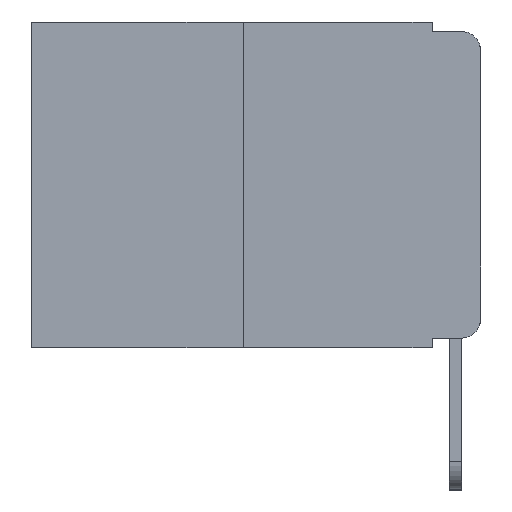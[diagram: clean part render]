
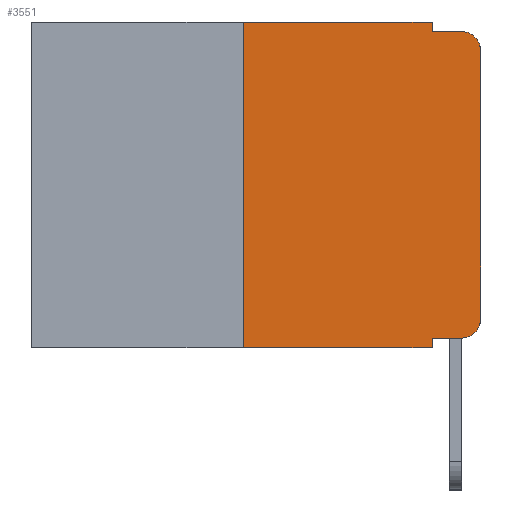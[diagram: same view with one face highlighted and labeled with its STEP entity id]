
A CAD part, left-side view. The second image highlights one B-rep face of the part: STEP entity #3551.
In plain terms, the highlighted planar face has unit normal (-1, 0, 0).
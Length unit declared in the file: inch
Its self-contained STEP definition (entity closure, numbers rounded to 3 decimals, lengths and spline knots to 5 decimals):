
#329 = CIRCLE ( 'NONE', #6323, 0.02 ) ;
#374 = VERTEX_POINT ( 'NONE', #1727 ) ;
#385 = EDGE_CURVE ( 'NONE', #7843, #9507, #11216, .T. ) ;
#397 = EDGE_CURVE ( 'NONE', #10086, #11016, #1003, .T. ) ;
#513 = EDGE_CURVE ( 'NONE', #4225, #12051, #2888, .T. ) ;
#934 = CARTESIAN_POINT ( 'NONE',  ( 0., 0.473, 0. ) ) ;
#1003 = LINE ( 'NONE', #11407, #8877 ) ;
#1082 = CARTESIAN_POINT ( 'NONE',  ( 0., 0.051, -0.333 ) ) ;
#1257 = CARTESIAN_POINT ( 'NONE',  ( 0., 0.25, 0. ) ) ;
#1320 = DIRECTION ( 'NONE',  ( 0., -1., 0. ) ) ;
#1373 = ORIENTED_EDGE ( 'NONE', *, *, #12733, .F. ) ;
#1403 = CARTESIAN_POINT ( 'NONE',  ( 0., 0.25, -0.343 ) ) ;
#1406 = VECTOR ( 'NONE', #1320, 39.37008 ) ;
#1475 = EDGE_CURVE ( 'NONE', #6086, #6269, #4521, .T. ) ;
#1726 = CARTESIAN_POINT ( 'NONE',  ( 0., 0.02, -0.313 ) ) ;
#1727 = CARTESIAN_POINT ( 'NONE',  ( 0., 0., -0.313 ) ) ;
#1803 = DIRECTION ( 'NONE',  ( 0., -1., 0. ) ) ;
#1959 = CARTESIAN_POINT ( 'NONE',  ( 0., 0.051, 0. ) ) ;
#2044 = ORIENTED_EDGE ( 'NONE', *, *, #513, .F. ) ;
#2200 = EDGE_CURVE ( 'NONE', #374, #6086, #4345, .T. ) ;
#2571 = DIRECTION ( 'NONE',  ( 0., 0., -1. ) ) ;
#2708 = DIRECTION ( 'NONE',  ( 0., 0., 1. ) ) ;
#2744 = ORIENTED_EDGE ( 'NONE', *, *, #4756, .F. ) ;
#2835 = DIRECTION ( 'NONE',  ( 0., 0., -1. ) ) ;
#2888 = LINE ( 'NONE', #11461, #12442 ) ;
#2893 = VERTEX_POINT ( 'NONE', #5303 ) ;
#3018 = CARTESIAN_POINT ( 'NONE',  ( 0., 0.02, -0.01 ) ) ;
#3077 = ORIENTED_EDGE ( 'NONE', *, *, #385, .T. ) ;
#3533 = LINE ( 'NONE', #1257, #8553 ) ;
#3551 = ADVANCED_FACE ( 'NONE', ( #6378 ), #11992, .F. ) ;
#4225 = VERTEX_POINT ( 'NONE', #11746 ) ;
#4344 = CARTESIAN_POINT ( 'NONE',  ( 0., 0.051, -0.333 ) ) ;
#4345 = LINE ( 'NONE', #6865, #11883 ) ;
#4492 = CARTESIAN_POINT ( 'NONE',  ( 0., 0.051, 0. ) ) ;
#4521 = CIRCLE ( 'NONE', #12044, 0.02 ) ;
#4611 = DIRECTION ( 'NONE',  ( 1., 0., 0. ) ) ;
#4756 = EDGE_CURVE ( 'NONE', #7843, #11016, #8027, .T. ) ;
#4771 = LINE ( 'NONE', #1959, #9944 ) ;
#5303 = CARTESIAN_POINT ( 'NONE',  ( 0., 0.051, -0.01 ) ) ;
#5332 = AXIS2_PLACEMENT_3D ( 'NONE', #934, #4611, #11715 ) ;
#5363 = VECTOR ( 'NONE', #2571, 39.37008 ) ;
#5385 = CARTESIAN_POINT ( 'NONE',  ( 0., 0.051, -0.343 ) ) ;
#5484 = DIRECTION ( 'NONE',  ( 0., 0., 1. ) ) ;
#6086 = VERTEX_POINT ( 'NONE', #11418 ) ;
#6137 = ORIENTED_EDGE ( 'NONE', *, *, #11921, .T. ) ;
#6269 = VERTEX_POINT ( 'NONE', #3018 ) ;
#6323 = AXIS2_PLACEMENT_3D ( 'NONE', #1726, #8865, #2835 ) ;
#6378 = FACE_OUTER_BOUND ( 'NONE', #11379, .T. ) ;
#6557 = CARTESIAN_POINT ( 'NONE',  ( 0., 0.051, -0.01 ) ) ;
#6865 = CARTESIAN_POINT ( 'NONE',  ( 0., 0., 0. ) ) ;
#7325 = DIRECTION ( 'NONE',  ( 0., -1., 0. ) ) ;
#7843 = VERTEX_POINT ( 'NONE', #1082 ) ;
#8027 = LINE ( 'NONE', #4492, #5363 ) ;
#8553 = VECTOR ( 'NONE', #5484, 39.37008 ) ;
#8748 = EDGE_CURVE ( 'NONE', #10086, #4225, #3533, .T. ) ;
#8865 = DIRECTION ( 'NONE',  ( -1., 0., 0. ) ) ;
#8877 = VECTOR ( 'NONE', #1803, 39.37008 ) ;
#8884 = ORIENTED_EDGE ( 'NONE', *, *, #1475, .T. ) ;
#9075 = DIRECTION ( 'NONE',  ( 0., 0., -1. ) ) ;
#9462 = ORIENTED_EDGE ( 'NONE', *, *, #10416, .F. ) ;
#9507 = VERTEX_POINT ( 'NONE', #10548 ) ;
#9944 = VECTOR ( 'NONE', #9075, 39.37008 ) ;
#10034 = ORIENTED_EDGE ( 'NONE', *, *, #8748, .F. ) ;
#10086 = VERTEX_POINT ( 'NONE', #1403 ) ;
#10416 = EDGE_CURVE ( 'NONE', #12051, #2893, #4771, .T. ) ;
#10548 = CARTESIAN_POINT ( 'NONE',  ( 0., 0.02, -0.333 ) ) ;
#10698 = ORIENTED_EDGE ( 'NONE', *, *, #2200, .T. ) ;
#10947 = VECTOR ( 'NONE', #7325, 39.37008 ) ;
#11016 = VERTEX_POINT ( 'NONE', #5385 ) ;
#11216 = LINE ( 'NONE', #4344, #10947 ) ;
#11379 = EDGE_LOOP ( 'NONE', ( #10698, #8884, #1373, #9462, #2044, #10034, #12320, #2744, #3077, #6137 ) ) ;
#11407 = CARTESIAN_POINT ( 'NONE',  ( 0., 0.473, -0.343 ) ) ;
#11418 = CARTESIAN_POINT ( 'NONE',  ( 0., 0., -0.03 ) ) ;
#11461 = CARTESIAN_POINT ( 'NONE',  ( 0., 0.473, 0. ) ) ;
#11490 = DIRECTION ( 'NONE',  ( 0., 0., -1. ) ) ;
#11585 = DIRECTION ( 'NONE',  ( -1., 0., 0. ) ) ;
#11715 = DIRECTION ( 'NONE',  ( 0., 0., -1. ) ) ;
#11746 = CARTESIAN_POINT ( 'NONE',  ( 0., 0.25, 0. ) ) ;
#11780 = CARTESIAN_POINT ( 'NONE',  ( 0., 0.02, -0.03 ) ) ;
#11812 = LINE ( 'NONE', #6557, #1406 ) ;
#11883 = VECTOR ( 'NONE', #2708, 39.37008 ) ;
#11921 = EDGE_CURVE ( 'NONE', #9507, #374, #329, .T. ) ;
#11983 = DIRECTION ( 'NONE',  ( 0., -1., 0. ) ) ;
#11992 = PLANE ( 'NONE',  #5332 ) ;
#12044 = AXIS2_PLACEMENT_3D ( 'NONE', #11780, #11585, #11490 ) ;
#12051 = VERTEX_POINT ( 'NONE', #12544 ) ;
#12320 = ORIENTED_EDGE ( 'NONE', *, *, #397, .T. ) ;
#12442 = VECTOR ( 'NONE', #11983, 39.37008 ) ;
#12544 = CARTESIAN_POINT ( 'NONE',  ( 0., 0.051, 0. ) ) ;
#12733 = EDGE_CURVE ( 'NONE', #2893, #6269, #11812, .T. ) ;
